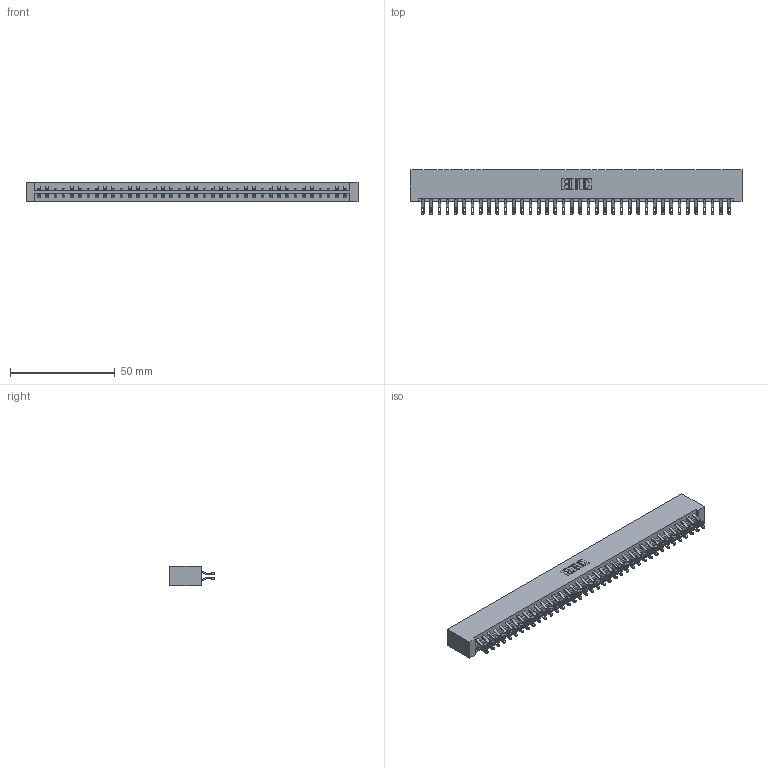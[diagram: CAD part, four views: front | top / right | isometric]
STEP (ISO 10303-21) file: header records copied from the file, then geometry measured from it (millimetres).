
FILE_DESCRIPTION (( 'STEP AP203' ), '1' );
FILE_NAME ('333-076-555-201.STEP', '2018-08-04T23:18:34', ( '' ), ( '' ), 'SwSTEP 2.0', 'SolidWorks 2016', '' );
FILE_SCHEMA (( 'CONFIG_CONTROL_DESIGN' ));
Length unit declared in the file: inch
Products named in the file (3): 345-292-001_555 Tail; 333-076-555-201; 333 Part_Lugless
Assembly tree (77 placements, depth 2):
  333-076-555-201
    333 Part_Lugless
    345-292-001_555 Tail  x76
Bounding box: 158.83 x 21.47 x 9.4 mm (x, y, z)
Volume: 17030.5 mm3; surface area: 20940.1 mm2
Topology: 77 solids, 77 shells, 4514 faces, 14195 edges, 9462 vertices
Faces by surface type: plane 2650, cylinder 1864
Entity records: 25013 total; most frequent: CARTESIAN_POINT 4184, ORIENTED_EDGE 4090, DIRECTION 3545, EDGE_CURVE 2045, VECTOR 1905, LINE 1905, VERTEX_POINT 1362, AXIS2_PLACEMENT_3D 820
